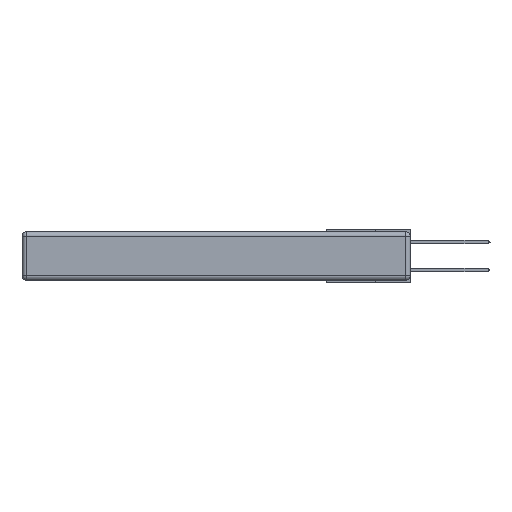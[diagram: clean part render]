
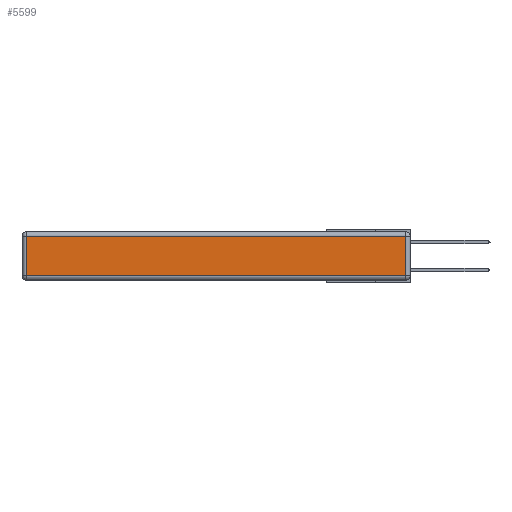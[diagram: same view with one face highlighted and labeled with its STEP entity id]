
A CAD part, left-side view. The second image highlights one B-rep face of the part: STEP entity #5599.
In plain terms, the highlighted planar face has unit normal (-1, 0, 0).
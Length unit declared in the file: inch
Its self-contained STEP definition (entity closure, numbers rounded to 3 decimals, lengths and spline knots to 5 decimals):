
#922 = VERTEX_POINT ( 'NONE', #10992 ) ;
#1459 = VECTOR ( 'NONE', #12278, 39.37008 ) ;
#2266 = CARTESIAN_POINT ( 'NONE',  ( 0., 0., -0.343 ) ) ;
#3872 = ORIENTED_EDGE ( 'NONE', *, *, #8970, .T. ) ;
#3885 = DIRECTION ( 'NONE',  ( 0., 1., 0. ) ) ;
#4764 = CARTESIAN_POINT ( 'NONE',  ( 0., 2.72, -0.03 ) ) ;
#4823 = PLANE ( 'NONE',  #11535 ) ;
#5445 = CARTESIAN_POINT ( 'NONE',  ( 0., 0., -0.313 ) ) ;
#5568 = LINE ( 'NONE', #5445, #14758 ) ;
#5599 = ADVANCED_FACE ( 'NONE', ( #7587 ), #4823, .T. ) ;
#5779 = CARTESIAN_POINT ( 'NONE',  ( 0., 2.72, -0.343 ) ) ;
#5871 = EDGE_CURVE ( 'NONE', #7184, #14285, #5568, .T. ) ;
#6389 = EDGE_CURVE ( 'NONE', #14285, #922, #14718, .T. ) ;
#6742 = DIRECTION ( 'NONE',  ( 0., -1., 0. ) ) ;
#6796 = CARTESIAN_POINT ( 'NONE',  ( 0., 0.03, -0.313 ) ) ;
#6950 = ORIENTED_EDGE ( 'NONE', *, *, #6389, .T. ) ;
#7184 = VERTEX_POINT ( 'NONE', #13274 ) ;
#7587 = FACE_OUTER_BOUND ( 'NONE', #10065, .T. ) ;
#8065 = VECTOR ( 'NONE', #15977, 39.37008 ) ;
#8379 = LINE ( 'NONE', #11907, #15876 ) ;
#8970 = EDGE_CURVE ( 'NONE', #922, #15712, #8379, .T. ) ;
#9185 = LINE ( 'NONE', #5779, #1459 ) ;
#10065 = EDGE_LOOP ( 'NONE', ( #13964, #6950, #3872, #10412 ) ) ;
#10412 = ORIENTED_EDGE ( 'NONE', *, *, #12774, .T. ) ;
#10992 = CARTESIAN_POINT ( 'NONE',  ( 0., 0.03, -0.03 ) ) ;
#11535 = AXIS2_PLACEMENT_3D ( 'NONE', #2266, #14203, #16727 ) ;
#11907 = CARTESIAN_POINT ( 'NONE',  ( 0., 2.75, -0.03 ) ) ;
#12278 = DIRECTION ( 'NONE',  ( 0., 0., -1. ) ) ;
#12774 = EDGE_CURVE ( 'NONE', #15712, #7184, #9185, .T. ) ;
#13274 = CARTESIAN_POINT ( 'NONE',  ( 0., 2.72, -0.313 ) ) ;
#13281 = CARTESIAN_POINT ( 'NONE',  ( 0., 0.03, -0.343 ) ) ;
#13964 = ORIENTED_EDGE ( 'NONE', *, *, #5871, .T. ) ;
#14203 = DIRECTION ( 'NONE',  ( -1., 0., 0. ) ) ;
#14285 = VERTEX_POINT ( 'NONE', #6796 ) ;
#14718 = LINE ( 'NONE', #13281, #8065 ) ;
#14758 = VECTOR ( 'NONE', #6742, 39.37008 ) ;
#15712 = VERTEX_POINT ( 'NONE', #4764 ) ;
#15876 = VECTOR ( 'NONE', #3885, 39.37008 ) ;
#15977 = DIRECTION ( 'NONE',  ( 0., 0., 1. ) ) ;
#16727 = DIRECTION ( 'NONE',  ( 0., 0., 1. ) ) ;
